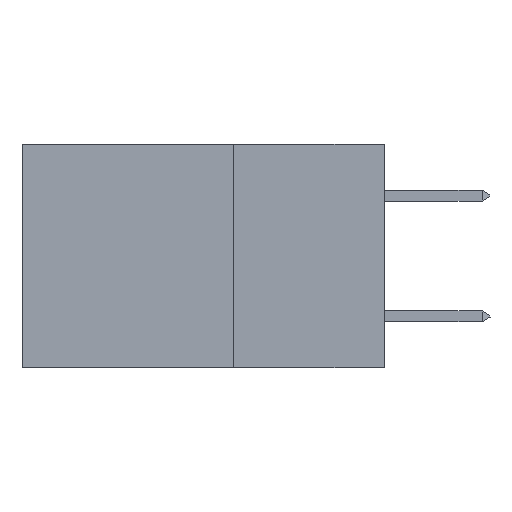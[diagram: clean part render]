
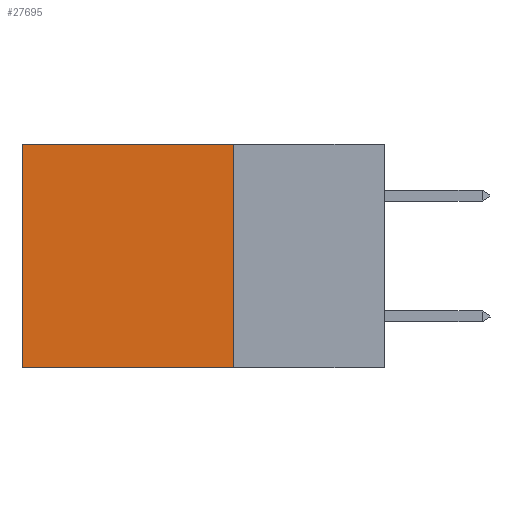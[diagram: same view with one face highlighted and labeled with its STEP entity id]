
A CAD part, left-side view. The second image highlights one B-rep face of the part: STEP entity #27695.
In plain terms, the highlighted planar face has unit normal (-1, 0, 0).
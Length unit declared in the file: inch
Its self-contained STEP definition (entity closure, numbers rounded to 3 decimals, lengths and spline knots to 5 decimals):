
#483 = DIRECTION ( 'NONE',  ( 0., 1., 0. ) ) ;
#791 = CARTESIAN_POINT ( 'NONE',  ( 0.2875, 0.6, -0.37 ) ) ;
#1604 = CARTESIAN_POINT ( 'NONE',  ( 0.2875, 0.25, 0. ) ) ;
#2069 = EDGE_LOOP ( 'NONE', ( #20879, #7753, #14071, #29859 ) ) ;
#3829 = EDGE_CURVE ( 'NONE', #14454, #25355, #6282, .T. ) ;
#4904 = LINE ( 'NONE', #34864, #23355 ) ;
#6282 = LINE ( 'NONE', #17679, #21287 ) ;
#6880 = PLANE ( 'NONE',  #8967 ) ;
#7753 = ORIENTED_EDGE ( 'NONE', *, *, #31551, .F. ) ;
#8967 = AXIS2_PLACEMENT_3D ( 'NONE', #22590, #31731, #16081 ) ;
#11026 = CARTESIAN_POINT ( 'NONE',  ( 0.2875, 0.25, -0.37 ) ) ;
#12437 = CARTESIAN_POINT ( 'NONE',  ( 0.2875, 0.6, 0. ) ) ;
#13045 = VERTEX_POINT ( 'NONE', #11026 ) ;
#13465 = LINE ( 'NONE', #33576, #14461 ) ;
#14071 = ORIENTED_EDGE ( 'NONE', *, *, #20183, .F. ) ;
#14454 = VERTEX_POINT ( 'NONE', #12437 ) ;
#14461 = VECTOR ( 'NONE', #21179, 39.37008 ) ;
#16081 = DIRECTION ( 'NONE',  ( 0., 0., -1. ) ) ;
#17679 = CARTESIAN_POINT ( 'NONE',  ( 0.2875, 0.6, 0. ) ) ;
#18047 = VERTEX_POINT ( 'NONE', #1604 ) ;
#20183 = EDGE_CURVE ( 'NONE', #18047, #13045, #13465, .T. ) ;
#20192 = FACE_OUTER_BOUND ( 'NONE', #2069, .T. ) ;
#20879 = ORIENTED_EDGE ( 'NONE', *, *, #3829, .T. ) ;
#21179 = DIRECTION ( 'NONE',  ( 0., 0., -1. ) ) ;
#21287 = VECTOR ( 'NONE', #39463, 39.37008 ) ;
#22590 = CARTESIAN_POINT ( 'NONE',  ( 0.2875, 0.25, 0. ) ) ;
#23355 = VECTOR ( 'NONE', #483, 39.37008 ) ;
#23882 = EDGE_CURVE ( 'NONE', #18047, #14454, #4904, .T. ) ;
#25355 = VERTEX_POINT ( 'NONE', #791 ) ;
#27695 = ADVANCED_FACE ( 'NONE', ( #20192 ), #6880, .F. ) ;
#27717 = VECTOR ( 'NONE', #36749, 39.37008 ) ;
#29859 = ORIENTED_EDGE ( 'NONE', *, *, #23882, .T. ) ;
#31551 = EDGE_CURVE ( 'NONE', #13045, #25355, #35043, .T. ) ;
#31731 = DIRECTION ( 'NONE',  ( 1., 0., 0. ) ) ;
#33576 = CARTESIAN_POINT ( 'NONE',  ( 0.2875, 0.25, 0. ) ) ;
#34285 = CARTESIAN_POINT ( 'NONE',  ( 0.2875, 0.25, -0.37 ) ) ;
#34864 = CARTESIAN_POINT ( 'NONE',  ( 0.2875, 0.25, 0. ) ) ;
#35043 = LINE ( 'NONE', #34285, #27717 ) ;
#36749 = DIRECTION ( 'NONE',  ( 0., 1., 0. ) ) ;
#39463 = DIRECTION ( 'NONE',  ( 0., 0., -1. ) ) ;
